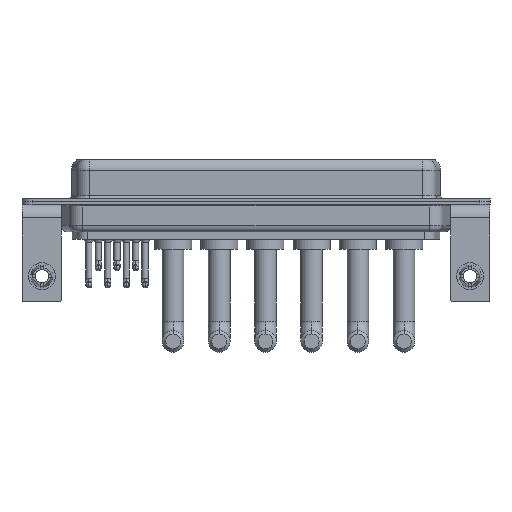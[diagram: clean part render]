
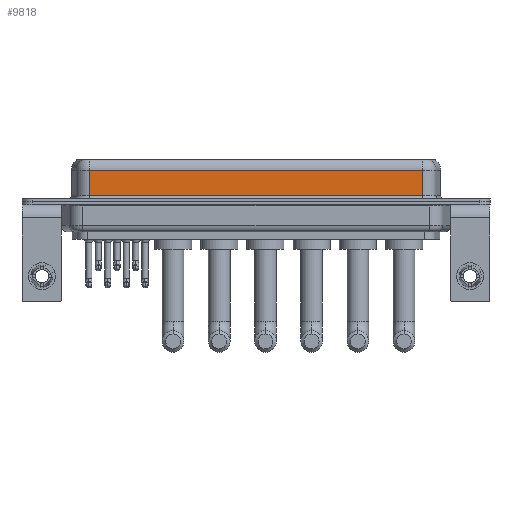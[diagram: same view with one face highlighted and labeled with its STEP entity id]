
A CAD part, front view. The second image highlights one B-rep face of the part: STEP entity #9818.
In plain terms, the highlighted planar face has unit normal (0, -1, 0).
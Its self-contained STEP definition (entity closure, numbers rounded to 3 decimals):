
#1015 = VECTOR ( 'NONE', #3966, 1000. ) ;
#1055 = CARTESIAN_POINT ( 'NONE',  ( 56.462, -3.95, 0.9 ) ) ;
#1410 = PLANE ( 'NONE',  #13003 ) ;
#2420 = VECTOR ( 'NONE', #12177, 1000. ) ;
#2441 = LINE ( 'NONE', #1055, #2420 ) ;
#2560 = DIRECTION ( 'NONE',  ( 0., 0., -1. ) ) ;
#3490 = EDGE_CURVE ( 'NONE', #15089, #18357, #2441, .T. ) ;
#3966 = DIRECTION ( 'NONE',  ( -1., 0., 0. ) ) ;
#6684 = VECTOR ( 'NONE', #15314, 1000. ) ;
#7859 = CARTESIAN_POINT ( 'NONE',  ( 7.038, -3.95, 0.9 ) ) ;
#7872 = CARTESIAN_POINT ( 'NONE',  ( 56.462, -3.95, 6.4 ) ) ;
#8034 = EDGE_LOOP ( 'NONE', ( #17859, #9518, #13585, #9292 ) ) ;
#9292 = ORIENTED_EDGE ( 'NONE', *, *, #3490, .T. ) ;
#9518 = ORIENTED_EDGE ( 'NONE', *, *, #16250, .T. ) ;
#9818 = ADVANCED_FACE ( 'NONE', ( #19090 ), #1410, .F. ) ;
#10062 = CARTESIAN_POINT ( 'NONE',  ( 7.038, -3.95, 4.65 ) ) ;
#10365 = CARTESIAN_POINT ( 'NONE',  ( 56.462, -3.95, 6.4 ) ) ;
#10422 = LINE ( 'NONE', #19860, #1015 ) ;
#11364 = EDGE_CURVE ( 'NONE', #16753, #15089, #13864, .T. ) ;
#11533 = VERTEX_POINT ( 'NONE', #15535 ) ;
#12177 = DIRECTION ( 'NONE',  ( 1., 0., 0. ) ) ;
#12722 = DIRECTION ( 'NONE',  ( 0., 0., 1. ) ) ;
#13003 = AXIS2_PLACEMENT_3D ( 'NONE', #7872, #20666, #12722 ) ;
#13418 = LINE ( 'NONE', #10365, #6684 ) ;
#13585 = ORIENTED_EDGE ( 'NONE', *, *, #11364, .T. ) ;
#13864 = LINE ( 'NONE', #20027, #18038 ) ;
#13975 = EDGE_CURVE ( 'NONE', #11533, #18357, #13418, .T. ) ;
#15089 = VERTEX_POINT ( 'NONE', #7859 ) ;
#15314 = DIRECTION ( 'NONE',  ( 0., 0., -1. ) ) ;
#15535 = CARTESIAN_POINT ( 'NONE',  ( 56.462, -3.95, 4.65 ) ) ;
#15933 = CARTESIAN_POINT ( 'NONE',  ( 56.462, -3.95, 0.9 ) ) ;
#16250 = EDGE_CURVE ( 'NONE', #11533, #16753, #10422, .T. ) ;
#16753 = VERTEX_POINT ( 'NONE', #10062 ) ;
#17859 = ORIENTED_EDGE ( 'NONE', *, *, #13975, .F. ) ;
#18038 = VECTOR ( 'NONE', #2560, 1000. ) ;
#18357 = VERTEX_POINT ( 'NONE', #15933 ) ;
#19090 = FACE_OUTER_BOUND ( 'NONE', #8034, .T. ) ;
#19860 = CARTESIAN_POINT ( 'NONE',  ( 56.462, -3.95, 4.65 ) ) ;
#20027 = CARTESIAN_POINT ( 'NONE',  ( 7.038, -3.95, 6.4 ) ) ;
#20666 = DIRECTION ( 'NONE',  ( 0., 1., 0. ) ) ;
